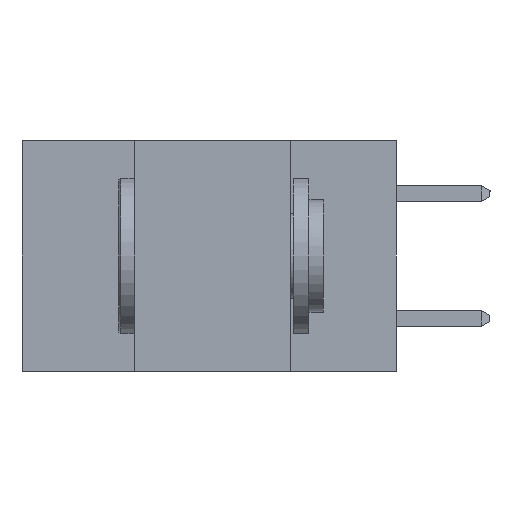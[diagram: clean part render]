
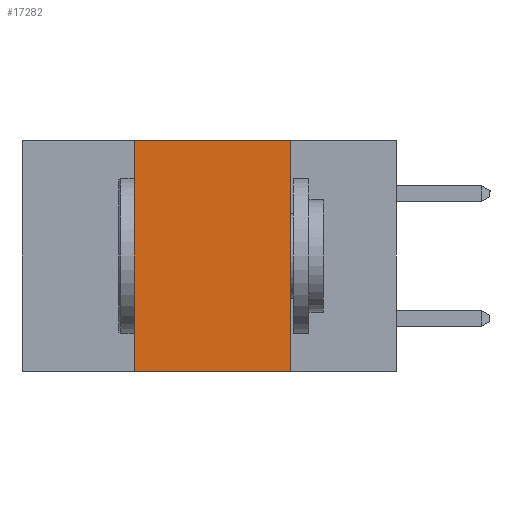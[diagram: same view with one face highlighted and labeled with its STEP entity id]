
A CAD part, left-side view. The second image highlights one B-rep face of the part: STEP entity #17282.
In plain terms, the highlighted planar face has unit normal (-1, 0, 0).
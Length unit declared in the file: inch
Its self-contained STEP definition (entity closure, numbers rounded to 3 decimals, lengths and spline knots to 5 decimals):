
#1554 = VERTEX_POINT ( 'NONE', #11456 ) ;
#2815 = ORIENTED_EDGE ( 'NONE', *, *, #23735, .F. ) ;
#3152 = PLANE ( 'NONE',  #22907 ) ;
#3958 = ORIENTED_EDGE ( 'NONE', *, *, #9735, .F. ) ;
#4704 = CARTESIAN_POINT ( 'NONE',  ( 0., 0.42, -0.37 ) ) ;
#5099 = DIRECTION ( 'NONE',  ( 0., -1., 0. ) ) ;
#5265 = ORIENTED_EDGE ( 'NONE', *, *, #19096, .T. ) ;
#5341 = CARTESIAN_POINT ( 'NONE',  ( 0., 0.42, -0.37 ) ) ;
#5440 = EDGE_LOOP ( 'NONE', ( #2815, #3958, #12965, #5265 ) ) ;
#6456 = CARTESIAN_POINT ( 'NONE',  ( 0., 0.17, -0.37 ) ) ;
#6850 = VERTEX_POINT ( 'NONE', #6456 ) ;
#6868 = VECTOR ( 'NONE', #18127, 39.37008 ) ;
#7513 = VECTOR ( 'NONE', #22177, 39.37008 ) ;
#8658 = CARTESIAN_POINT ( 'NONE',  ( 0., 0.6, 0. ) ) ;
#9140 = CARTESIAN_POINT ( 'NONE',  ( 0., 0.17, 0. ) ) ;
#9263 = LINE ( 'NONE', #5341, #7513 ) ;
#9735 = EDGE_CURVE ( 'NONE', #1554, #21256, #14573, .T. ) ;
#10160 = CARTESIAN_POINT ( 'NONE',  ( 0., 0.6, 0. ) ) ;
#10401 = DIRECTION ( 'NONE',  ( 0., 0., -1. ) ) ;
#10667 = CARTESIAN_POINT ( 'NONE',  ( 0., 0.17, -0.37 ) ) ;
#10901 = LINE ( 'NONE', #10667, #14324 ) ;
#11456 = CARTESIAN_POINT ( 'NONE',  ( 0., 0.42, 0. ) ) ;
#12965 = ORIENTED_EDGE ( 'NONE', *, *, #14618, .F. ) ;
#14324 = VECTOR ( 'NONE', #22096, 39.37008 ) ;
#14573 = LINE ( 'NONE', #8658, #23898 ) ;
#14618 = EDGE_CURVE ( 'NONE', #17763, #1554, #9263, .T. ) ;
#16087 = DIRECTION ( 'NONE',  ( 1., 0., 0. ) ) ;
#17282 = ADVANCED_FACE ( 'NONE', ( #23192 ), #3152, .F. ) ;
#17650 = CARTESIAN_POINT ( 'NONE',  ( 0., 0.6, -0.37 ) ) ;
#17763 = VERTEX_POINT ( 'NONE', #4704 ) ;
#18127 = DIRECTION ( 'NONE',  ( 0., -1., 0. ) ) ;
#19096 = EDGE_CURVE ( 'NONE', #17763, #6850, #21820, .T. ) ;
#21256 = VERTEX_POINT ( 'NONE', #9140 ) ;
#21820 = LINE ( 'NONE', #17650, #6868 ) ;
#22096 = DIRECTION ( 'NONE',  ( 0., 0., -1. ) ) ;
#22177 = DIRECTION ( 'NONE',  ( 0., 0., 1. ) ) ;
#22907 = AXIS2_PLACEMENT_3D ( 'NONE', #10160, #16087, #10401 ) ;
#23192 = FACE_OUTER_BOUND ( 'NONE', #5440, .T. ) ;
#23735 = EDGE_CURVE ( 'NONE', #21256, #6850, #10901, .T. ) ;
#23898 = VECTOR ( 'NONE', #5099, 39.37008 ) ;
